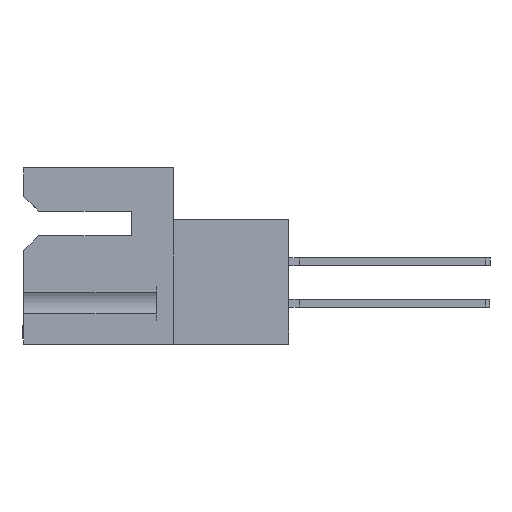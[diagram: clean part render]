
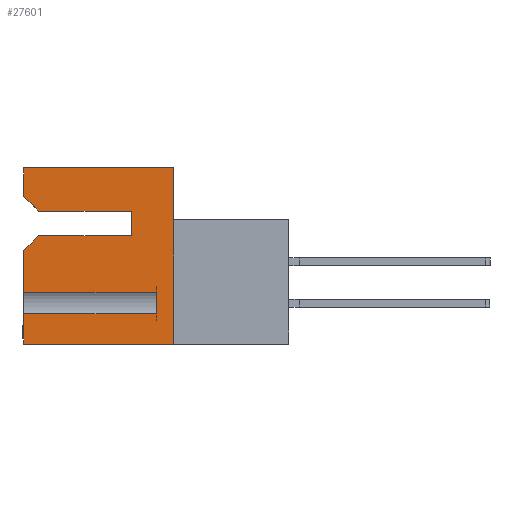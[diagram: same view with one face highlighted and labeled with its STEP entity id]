
A CAD part, left-side view. The second image highlights one B-rep face of the part: STEP entity #27601.
In plain terms, the highlighted planar face has unit normal (-1, 0, 0).
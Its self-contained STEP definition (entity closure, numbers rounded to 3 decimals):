
#298 = EDGE_CURVE ( 'NONE', #38200, #40669, #4373, .T. ) ;
#990 = ORIENTED_EDGE ( 'NONE', *, *, #13063, .F. ) ;
#1330 = CARTESIAN_POINT ( 'NONE',  ( 0., 10.363, -5.182 ) ) ;
#1747 = VERTEX_POINT ( 'NONE', #33789 ) ;
#2616 = EDGE_CURVE ( 'NONE', #45216, #20670, #25285, .T. ) ;
#2784 = LINE ( 'NONE', #33461, #27716 ) ;
#2806 = CARTESIAN_POINT ( 'NONE',  ( 0., 1.346, -9.556 ) ) ;
#3012 = EDGE_CURVE ( 'NONE', #30114, #32673, #18624, .T. ) ;
#3616 = CARTESIAN_POINT ( 'NONE',  ( 0., 3.251, -5.182 ) ) ;
#3630 = VECTOR ( 'NONE', #7373, 1000. ) ;
#4154 = AXIS2_PLACEMENT_3D ( 'NONE', #19139, #12628, #30583 ) ;
#4373 = LINE ( 'NONE', #27600, #12691 ) ;
#4663 = CARTESIAN_POINT ( 'NONE',  ( 0., 3.251, -5.182 ) ) ;
#5249 = CARTESIAN_POINT ( 'NONE',  ( 0., 11.506, -11.17 ) ) ;
#5694 = CARTESIAN_POINT ( 'NONE',  ( 0., 1.346, -11.17 ) ) ;
#6157 = VERTEX_POINT ( 'NONE', #29554 ) ;
#6548 = ORIENTED_EDGE ( 'NONE', *, *, #28926, .F. ) ;
#6833 = DIRECTION ( 'NONE',  ( 0., 0., -1. ) ) ;
#7373 = DIRECTION ( 'NONE',  ( 0., -0.707, -0.707 ) ) ;
#8311 = LINE ( 'NONE', #1330, #28270 ) ;
#9041 = CARTESIAN_POINT ( 'NONE',  ( 0., 11.506, 0. ) ) ;
#9308 = ORIENTED_EDGE ( 'NONE', *, *, #11925, .F. ) ;
#9487 = ORIENTED_EDGE ( 'NONE', *, *, #14809, .F. ) ;
#9591 = EDGE_CURVE ( 'NONE', #35257, #24309, #33819, .T. ) ;
#9752 = CARTESIAN_POINT ( 'NONE',  ( 0., 10.363, -5.182 ) ) ;
#10269 = LINE ( 'NONE', #3616, #31327 ) ;
#10826 = CARTESIAN_POINT ( 'NONE',  ( 0., 11.506, -13.487 ) ) ;
#10883 = ORIENTED_EDGE ( 'NONE', *, *, #32350, .F. ) ;
#11604 = DIRECTION ( 'NONE',  ( 0., -1., 0. ) ) ;
#11925 = EDGE_CURVE ( 'NONE', #6157, #38200, #17023, .T. ) ;
#12101 = LINE ( 'NONE', #19486, #23723 ) ;
#12520 = DIRECTION ( 'NONE',  ( 0., 1., 0. ) ) ;
#12628 = DIRECTION ( 'NONE',  ( 1., 0., 0. ) ) ;
#12691 = VECTOR ( 'NONE', #6833, 1000. ) ;
#13063 = EDGE_CURVE ( 'NONE', #20670, #38591, #10269, .T. ) ;
#13276 = EDGE_CURVE ( 'NONE', #45216, #27538, #8311, .T. ) ;
#13389 = EDGE_LOOP ( 'NONE', ( #9487, #27082, #9308, #45513, #35092, #6548, #990, #17573, #19608, #38505, #21269, #16927, #35597, #10883 ) ) ;
#13402 = CARTESIAN_POINT ( 'NONE',  ( 0., 11.506, -13.487 ) ) ;
#13731 = CARTESIAN_POINT ( 'NONE',  ( 0., 11.506, -13.487 ) ) ;
#14430 = LINE ( 'NONE', #38417, #17749 ) ;
#14702 = DIRECTION ( 'NONE',  ( 0., 0., 1. ) ) ;
#14809 = EDGE_CURVE ( 'NONE', #40669, #1747, #12101, .T. ) ;
#15528 = CARTESIAN_POINT ( 'NONE',  ( 0., 11.506, -9.556 ) ) ;
#16927 = ORIENTED_EDGE ( 'NONE', *, *, #26990, .F. ) ;
#17023 = LINE ( 'NONE', #9041, #32545 ) ;
#17573 = ORIENTED_EDGE ( 'NONE', *, *, #2616, .F. ) ;
#17749 = VECTOR ( 'NONE', #45683, 1000. ) ;
#18624 = LINE ( 'NONE', #32150, #3630 ) ;
#18879 = DIRECTION ( 'NONE',  ( 0., 0., 1. ) ) ;
#19139 = CARTESIAN_POINT ( 'NONE',  ( 0., 0., 0. ) ) ;
#19486 = CARTESIAN_POINT ( 'NONE',  ( 0., -8.814, -13.487 ) ) ;
#19608 = ORIENTED_EDGE ( 'NONE', *, *, #13276, .T. ) ;
#20670 = VERTEX_POINT ( 'NONE', #4663 ) ;
#21269 = ORIENTED_EDGE ( 'NONE', *, *, #26340, .T. ) ;
#22144 = DIRECTION ( 'NONE',  ( 0., 1., 0. ) ) ;
#23479 = DIRECTION ( 'NONE',  ( 0., 1., 0. ) ) ;
#23723 = VECTOR ( 'NONE', #23479, 1000. ) ;
#24309 = VERTEX_POINT ( 'NONE', #5249 ) ;
#24325 = VECTOR ( 'NONE', #12520, 1000. ) ;
#24949 = LINE ( 'NONE', #25557, #29402 ) ;
#25009 = DIRECTION ( 'NONE',  ( 0., 0., 1. ) ) ;
#25155 = VERTEX_POINT ( 'NONE', #15528 ) ;
#25285 = LINE ( 'NONE', #43371, #34220 ) ;
#25399 = LINE ( 'NONE', #13402, #35075 ) ;
#25557 = CARTESIAN_POINT ( 'NONE',  ( 0., 0., -3.302 ) ) ;
#26340 = EDGE_CURVE ( 'NONE', #25155, #37377, #14430, .T. ) ;
#26990 = EDGE_CURVE ( 'NONE', #35257, #37377, #2784, .T. ) ;
#27082 = ORIENTED_EDGE ( 'NONE', *, *, #298, .F. ) ;
#27472 = DIRECTION ( 'NONE',  ( 0., 0., 1. ) ) ;
#27538 = VERTEX_POINT ( 'NONE', #33411 ) ;
#27600 = CARTESIAN_POINT ( 'NONE',  ( 0., 0., 0. ) ) ;
#27601 = ADVANCED_FACE ( 'NONE', ( #44880 ), #40373, .F. ) ;
#27665 = DIRECTION ( 'NONE',  ( 0., 0., 1. ) ) ;
#27716 = VECTOR ( 'NONE', #18879, 1000. ) ;
#28270 = VECTOR ( 'NONE', #32807, 1000. ) ;
#28926 = EDGE_CURVE ( 'NONE', #38591, #32673, #24949, .T. ) ;
#29402 = VECTOR ( 'NONE', #22144, 1000. ) ;
#29554 = CARTESIAN_POINT ( 'NONE',  ( 0., 11.506, 0. ) ) ;
#29801 = CARTESIAN_POINT ( 'NONE',  ( 0., 10.363, -3.302 ) ) ;
#30114 = VERTEX_POINT ( 'NONE', #35239 ) ;
#30583 = DIRECTION ( 'NONE',  ( 0., 0., -1. ) ) ;
#31327 = VECTOR ( 'NONE', #25009, 1000. ) ;
#31380 = EDGE_CURVE ( 'NONE', #30114, #6157, #25399, .T. ) ;
#32150 = CARTESIAN_POINT ( 'NONE',  ( 0., 10.363, -3.302 ) ) ;
#32350 = EDGE_CURVE ( 'NONE', #1747, #24309, #45040, .T. ) ;
#32545 = VECTOR ( 'NONE', #33713, 1000. ) ;
#32673 = VERTEX_POINT ( 'NONE', #29801 ) ;
#32807 = DIRECTION ( 'NONE',  ( 0., 0.707, -0.707 ) ) ;
#32892 = CARTESIAN_POINT ( 'NONE',  ( 0., 1.346, -11.17 ) ) ;
#33411 = CARTESIAN_POINT ( 'NONE',  ( 0., 11.506, -6.325 ) ) ;
#33461 = CARTESIAN_POINT ( 'NONE',  ( 0., 1.346, 0. ) ) ;
#33713 = DIRECTION ( 'NONE',  ( 0., -1., 0. ) ) ;
#33789 = CARTESIAN_POINT ( 'NONE',  ( 0., 11.506, -13.487 ) ) ;
#33819 = LINE ( 'NONE', #5694, #24325 ) ;
#34220 = VECTOR ( 'NONE', #11604, 1000. ) ;
#34486 = CARTESIAN_POINT ( 'NONE',  ( 0., 0., -13.487 ) ) ;
#34535 = EDGE_CURVE ( 'NONE', #25155, #27538, #37080, .T. ) ;
#35075 = VECTOR ( 'NONE', #27472, 1000. ) ;
#35092 = ORIENTED_EDGE ( 'NONE', *, *, #3012, .T. ) ;
#35239 = CARTESIAN_POINT ( 'NONE',  ( 0., 11.506, -2.159 ) ) ;
#35257 = VERTEX_POINT ( 'NONE', #32892 ) ;
#35596 = VECTOR ( 'NONE', #27665, 1000. ) ;
#35597 = ORIENTED_EDGE ( 'NONE', *, *, #9591, .T. ) ;
#37080 = LINE ( 'NONE', #10826, #39832 ) ;
#37377 = VERTEX_POINT ( 'NONE', #2806 ) ;
#38200 = VERTEX_POINT ( 'NONE', #39768 ) ;
#38417 = CARTESIAN_POINT ( 'NONE',  ( 0., 1.346, -9.556 ) ) ;
#38505 = ORIENTED_EDGE ( 'NONE', *, *, #34535, .F. ) ;
#38591 = VERTEX_POINT ( 'NONE', #42344 ) ;
#39768 = CARTESIAN_POINT ( 'NONE',  ( 0., 0., 0. ) ) ;
#39832 = VECTOR ( 'NONE', #14702, 1000. ) ;
#40373 = PLANE ( 'NONE',  #4154 ) ;
#40669 = VERTEX_POINT ( 'NONE', #34486 ) ;
#42344 = CARTESIAN_POINT ( 'NONE',  ( 0., 3.251, -3.302 ) ) ;
#43371 = CARTESIAN_POINT ( 'NONE',  ( 0., 0., -5.182 ) ) ;
#44880 = FACE_OUTER_BOUND ( 'NONE', #13389, .T. ) ;
#45040 = LINE ( 'NONE', #13731, #35596 ) ;
#45216 = VERTEX_POINT ( 'NONE', #9752 ) ;
#45513 = ORIENTED_EDGE ( 'NONE', *, *, #31380, .F. ) ;
#45683 = DIRECTION ( 'NONE',  ( 0., -1., 0. ) ) ;
